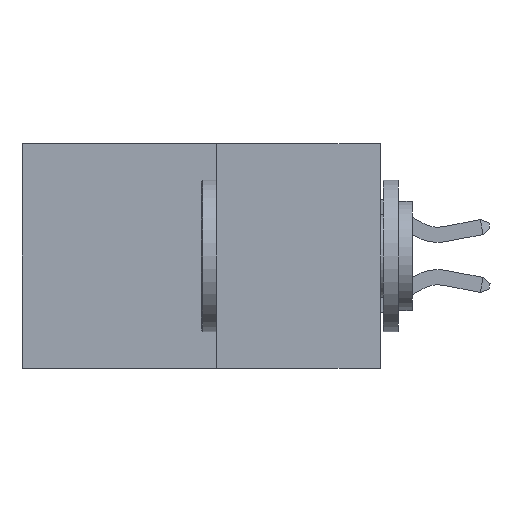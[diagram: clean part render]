
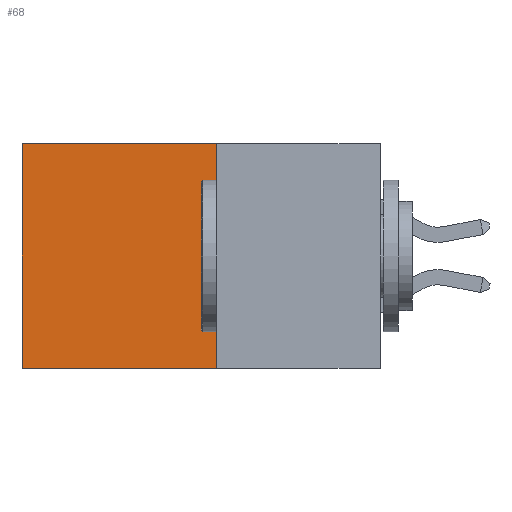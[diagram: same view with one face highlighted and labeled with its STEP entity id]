
A CAD part, left-side view. The second image highlights one B-rep face of the part: STEP entity #68.
In plain terms, the highlighted planar face has unit normal (-1, 0, 0).
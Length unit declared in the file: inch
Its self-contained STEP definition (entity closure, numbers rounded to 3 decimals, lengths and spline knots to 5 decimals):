
#68 = ADVANCED_FACE ( 'NONE', ( #9186 ), #7837, .F. ) ;
#330 = VERTEX_POINT ( 'NONE', #8157 ) ;
#348 = EDGE_CURVE ( 'NONE', #330, #8875, #4384, .T. ) ;
#1502 = LINE ( 'NONE', #2565, #3364 ) ;
#1686 = ORIENTED_EDGE ( 'NONE', *, *, #4222, .T. ) ;
#2240 = DIRECTION ( 'NONE',  ( 0., 1., 0. ) ) ;
#2269 = DIRECTION ( 'NONE',  ( 0., 0., -1. ) ) ;
#2271 = DIRECTION ( 'NONE',  ( 1., 0., 0. ) ) ;
#2565 = CARTESIAN_POINT ( 'NONE',  ( 0.277, 0.59, -0.37 ) ) ;
#2573 = VERTEX_POINT ( 'NONE', #9915 ) ;
#2985 = DIRECTION ( 'NONE',  ( 0., 0., -1. ) ) ;
#3205 = CARTESIAN_POINT ( 'NONE',  ( 0.277, 0.27, -0.37 ) ) ;
#3364 = VECTOR ( 'NONE', #2985, 39.37008 ) ;
#3429 = EDGE_CURVE ( 'NONE', #330, #2573, #9556, .T. ) ;
#3785 = VERTEX_POINT ( 'NONE', #6737 ) ;
#3951 = ORIENTED_EDGE ( 'NONE', *, *, #8779, .F. ) ;
#4222 = EDGE_CURVE ( 'NONE', #2573, #3785, #1502, .T. ) ;
#4305 = LINE ( 'NONE', #4710, #8287 ) ;
#4384 = LINE ( 'NONE', #6974, #10301 ) ;
#4473 = EDGE_LOOP ( 'NONE', ( #1686, #3951, #6121, #8211 ) ) ;
#4710 = CARTESIAN_POINT ( 'NONE',  ( 0.277, 0.27, -0.37 ) ) ;
#6121 = ORIENTED_EDGE ( 'NONE', *, *, #348, .F. ) ;
#6353 = AXIS2_PLACEMENT_3D ( 'NONE', #7509, #2271, #2269 ) ;
#6737 = CARTESIAN_POINT ( 'NONE',  ( 0.277, 0.59, -0.37 ) ) ;
#6974 = CARTESIAN_POINT ( 'NONE',  ( 0.277, 0.27, -0.37 ) ) ;
#7509 = CARTESIAN_POINT ( 'NONE',  ( 0.277, 0.27, -0.37 ) ) ;
#7553 = VECTOR ( 'NONE', #7786, 39.37008 ) ;
#7786 = DIRECTION ( 'NONE',  ( 0., 1., 0. ) ) ;
#7837 = PLANE ( 'NONE',  #6353 ) ;
#7873 = CARTESIAN_POINT ( 'NONE',  ( 0.277, 0.27, 0. ) ) ;
#8157 = CARTESIAN_POINT ( 'NONE',  ( 0.277, 0.27, 0. ) ) ;
#8211 = ORIENTED_EDGE ( 'NONE', *, *, #3429, .T. ) ;
#8287 = VECTOR ( 'NONE', #2240, 39.37008 ) ;
#8635 = DIRECTION ( 'NONE',  ( 0., 0., -1. ) ) ;
#8779 = EDGE_CURVE ( 'NONE', #8875, #3785, #4305, .T. ) ;
#8875 = VERTEX_POINT ( 'NONE', #3205 ) ;
#9186 = FACE_OUTER_BOUND ( 'NONE', #4473, .T. ) ;
#9556 = LINE ( 'NONE', #7873, #7553 ) ;
#9915 = CARTESIAN_POINT ( 'NONE',  ( 0.277, 0.59, 0. ) ) ;
#10301 = VECTOR ( 'NONE', #8635, 39.37008 ) ;
